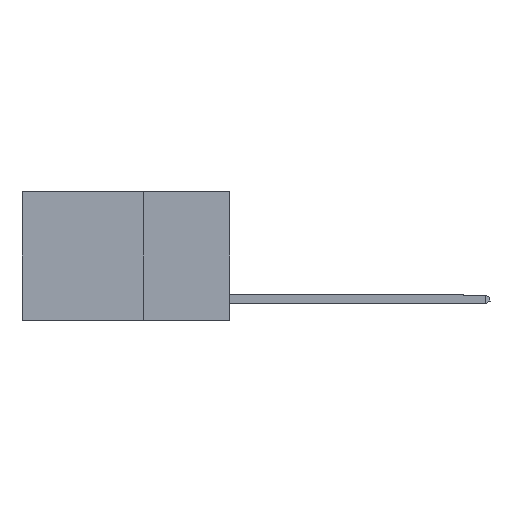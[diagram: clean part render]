
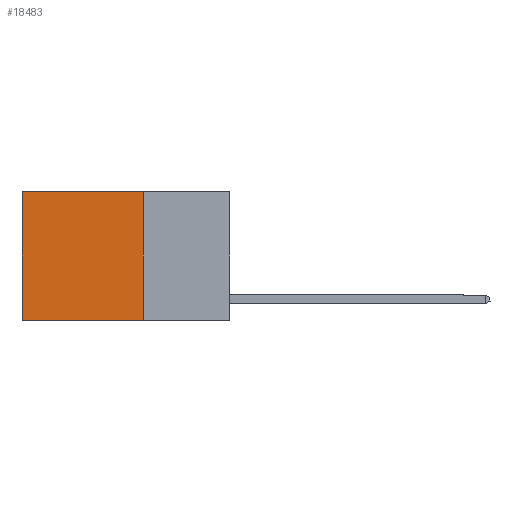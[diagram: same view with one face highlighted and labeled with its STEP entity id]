
A CAD part, left-side view. The second image highlights one B-rep face of the part: STEP entity #18483.
In plain terms, the highlighted planar face has unit normal (-1, 0, 0).
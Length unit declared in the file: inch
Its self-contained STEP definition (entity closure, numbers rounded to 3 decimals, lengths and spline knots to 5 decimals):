
#315 = VECTOR ( 'NONE', #14940, 39.37008 ) ;
#375 = ORIENTED_EDGE ( 'NONE', *, *, #9938, .T. ) ;
#2102 = DIRECTION ( 'NONE',  ( 1., 0., 0. ) ) ;
#2103 = DIRECTION ( 'NONE',  ( 0., 1., 0. ) ) ;
#2370 = CARTESIAN_POINT ( 'NONE',  ( 0.2625, 0.6, 0. ) ) ;
#3312 = ORIENTED_EDGE ( 'NONE', *, *, #4832, .F. ) ;
#3399 = ORIENTED_EDGE ( 'NONE', *, *, #16560, .T. ) ;
#3534 = EDGE_LOOP ( 'NONE', ( #375, #7466, #3312, #3399 ) ) ;
#3693 = VERTEX_POINT ( 'NONE', #19335 ) ;
#4832 = EDGE_CURVE ( 'NONE', #15447, #8712, #18336, .T. ) ;
#6049 = CARTESIAN_POINT ( 'NONE',  ( 0.2625, 0.6, 0. ) ) ;
#7465 = DIRECTION ( 'NONE',  ( 0., 1., 0. ) ) ;
#7466 = ORIENTED_EDGE ( 'NONE', *, *, #14008, .F. ) ;
#8712 = VERTEX_POINT ( 'NONE', #11517 ) ;
#8815 = VECTOR ( 'NONE', #11978, 39.37008 ) ;
#9419 = LINE ( 'NONE', #2370, #315 ) ;
#9938 = EDGE_CURVE ( 'NONE', #14141, #3693, #9419, .T. ) ;
#11517 = CARTESIAN_POINT ( 'NONE',  ( 0.2625, 0.25, -0.37 ) ) ;
#11720 = LINE ( 'NONE', #16398, #15899 ) ;
#11978 = DIRECTION ( 'NONE',  ( 0., 0., -1. ) ) ;
#12890 = CARTESIAN_POINT ( 'NONE',  ( 0.2625, 0.25, 0. ) ) ;
#12892 = CARTESIAN_POINT ( 'NONE',  ( 0.2625, 0.25, 0. ) ) ;
#13551 = LINE ( 'NONE', #12892, #22526 ) ;
#14008 = EDGE_CURVE ( 'NONE', #8712, #3693, #11720, .T. ) ;
#14141 = VERTEX_POINT ( 'NONE', #6049 ) ;
#14347 = AXIS2_PLACEMENT_3D ( 'NONE', #12890, #2102, #14663 ) ;
#14663 = DIRECTION ( 'NONE',  ( 0., 0., -1. ) ) ;
#14940 = DIRECTION ( 'NONE',  ( 0., 0., -1. ) ) ;
#15447 = VERTEX_POINT ( 'NONE', #16598 ) ;
#15899 = VECTOR ( 'NONE', #7465, 39.37008 ) ;
#16398 = CARTESIAN_POINT ( 'NONE',  ( 0.2625, 0.25, -0.37 ) ) ;
#16560 = EDGE_CURVE ( 'NONE', #15447, #14141, #13551, .T. ) ;
#16598 = CARTESIAN_POINT ( 'NONE',  ( 0.2625, 0.25, 0. ) ) ;
#18336 = LINE ( 'NONE', #20830, #8815 ) ;
#18483 = ADVANCED_FACE ( 'NONE', ( #19981 ), #21785, .F. ) ;
#19335 = CARTESIAN_POINT ( 'NONE',  ( 0.2625, 0.6, -0.37 ) ) ;
#19981 = FACE_OUTER_BOUND ( 'NONE', #3534, .T. ) ;
#20830 = CARTESIAN_POINT ( 'NONE',  ( 0.2625, 0.25, 0. ) ) ;
#21785 = PLANE ( 'NONE',  #14347 ) ;
#22526 = VECTOR ( 'NONE', #2103, 39.37008 ) ;
